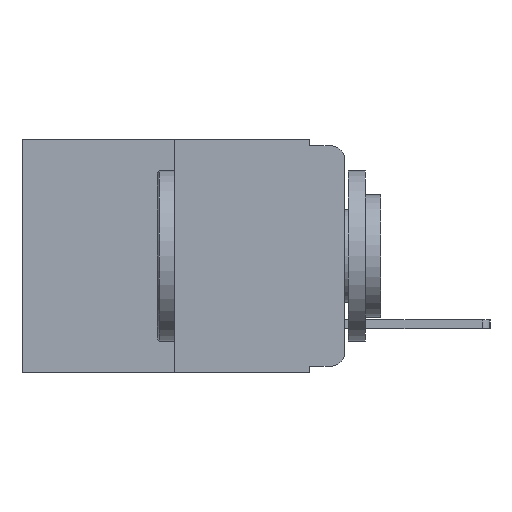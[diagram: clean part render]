
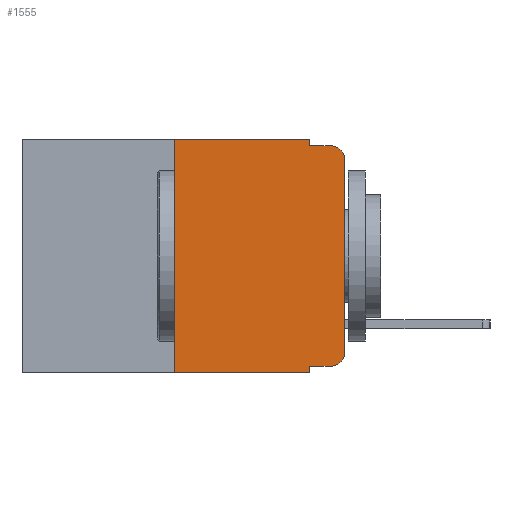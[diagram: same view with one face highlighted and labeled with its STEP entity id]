
A CAD part, left-side view. The second image highlights one B-rep face of the part: STEP entity #1555.
In plain terms, the highlighted planar face has unit normal (-1, 0, 0).
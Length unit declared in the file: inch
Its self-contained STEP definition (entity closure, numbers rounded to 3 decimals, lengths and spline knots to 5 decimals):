
#567 = AXIS2_PLACEMENT_3D ( 'NONE', #3577, #10929, #4782 ) ;
#870 = LINE ( 'NONE', #13710, #9405 ) ;
#1305 = LINE ( 'NONE', #6623, #4194 ) ;
#1432 = ORIENTED_EDGE ( 'NONE', *, *, #9063, .F. ) ;
#1555 = ADVANCED_FACE ( 'NONE', ( #7393 ), #8479, .F. ) ;
#1598 = VERTEX_POINT ( 'NONE', #12378 ) ;
#1655 = ORIENTED_EDGE ( 'NONE', *, *, #9168, .T. ) ;
#1799 = VERTEX_POINT ( 'NONE', #11805 ) ;
#1927 = CIRCLE ( 'NONE', #567, 0.02 ) ;
#2148 = LINE ( 'NONE', #9574, #10049 ) ;
#2835 = VECTOR ( 'NONE', #12388, 39.37008 ) ;
#3334 = CARTESIAN_POINT ( 'NONE',  ( 0., 0.051, -0.343 ) ) ;
#3475 = DIRECTION ( 'NONE',  ( 0., 0., -1. ) ) ;
#3577 = CARTESIAN_POINT ( 'NONE',  ( 0., 0.02, -0.313 ) ) ;
#3671 = DIRECTION ( 'NONE',  ( 0., 0., -1. ) ) ;
#3675 = DIRECTION ( 'NONE',  ( 1., 0., 0. ) ) ;
#4119 = CARTESIAN_POINT ( 'NONE',  ( 0., 0.473, 0. ) ) ;
#4194 = VECTOR ( 'NONE', #7621, 39.37008 ) ;
#4229 = CARTESIAN_POINT ( 'NONE',  ( 0., 0.051, 0. ) ) ;
#4305 = CARTESIAN_POINT ( 'NONE',  ( 0., 0.473, 0. ) ) ;
#4473 = CARTESIAN_POINT ( 'NONE',  ( 0., 0.02, -0.03 ) ) ;
#4632 = EDGE_CURVE ( 'NONE', #5760, #4680, #6195, .T. ) ;
#4680 = VERTEX_POINT ( 'NONE', #4229 ) ;
#4782 = DIRECTION ( 'NONE',  ( 0., 0., -1. ) ) ;
#4928 = CIRCLE ( 'NONE', #12534, 0.02 ) ;
#4971 = LINE ( 'NONE', #8127, #7082 ) ;
#5041 = VERTEX_POINT ( 'NONE', #12837 ) ;
#5429 = VECTOR ( 'NONE', #11841, 39.37008 ) ;
#5588 = DIRECTION ( 'NONE',  ( 0., 0., -1. ) ) ;
#5634 = DIRECTION ( 'NONE',  ( 0., 0., -1. ) ) ;
#5760 = VERTEX_POINT ( 'NONE', #13702 ) ;
#6060 = ORIENTED_EDGE ( 'NONE', *, *, #9047, .T. ) ;
#6081 = VECTOR ( 'NONE', #3475, 39.37008 ) ;
#6195 = LINE ( 'NONE', #4119, #2835 ) ;
#6409 = VECTOR ( 'NONE', #12736, 39.37008 ) ;
#6623 = CARTESIAN_POINT ( 'NONE',  ( 0., 0.051, -0.01 ) ) ;
#7048 = VERTEX_POINT ( 'NONE', #13305 ) ;
#7082 = VECTOR ( 'NONE', #9167, 39.37008 ) ;
#7393 = FACE_OUTER_BOUND ( 'NONE', #12363, .T. ) ;
#7621 = DIRECTION ( 'NONE',  ( 0., -1., 0. ) ) ;
#7659 = EDGE_CURVE ( 'NONE', #9181, #9071, #4971, .T. ) ;
#7700 = AXIS2_PLACEMENT_3D ( 'NONE', #4305, #3675, #3671 ) ;
#7748 = CARTESIAN_POINT ( 'NONE',  ( 0., 0.051, -0.333 ) ) ;
#7749 = ORIENTED_EDGE ( 'NONE', *, *, #7659, .T. ) ;
#8127 = CARTESIAN_POINT ( 'NONE',  ( 0., 0.473, -0.343 ) ) ;
#8351 = ORIENTED_EDGE ( 'NONE', *, *, #9111, .F. ) ;
#8479 = PLANE ( 'NONE',  #7700 ) ;
#9042 = EDGE_CURVE ( 'NONE', #1598, #5041, #2148, .T. ) ;
#9047 = EDGE_CURVE ( 'NONE', #5041, #7048, #4928, .T. ) ;
#9063 = EDGE_CURVE ( 'NONE', #11712, #7048, #1305, .T. ) ;
#9071 = VERTEX_POINT ( 'NONE', #3334 ) ;
#9111 = EDGE_CURVE ( 'NONE', #4680, #11712, #870, .T. ) ;
#9116 = EDGE_CURVE ( 'NONE', #9181, #5760, #11791, .T. ) ;
#9153 = ORIENTED_EDGE ( 'NONE', *, *, #9116, .F. ) ;
#9164 = EDGE_CURVE ( 'NONE', #13082, #9071, #13848, .T. ) ;
#9167 = DIRECTION ( 'NONE',  ( 0., -1., 0. ) ) ;
#9168 = EDGE_CURVE ( 'NONE', #13082, #1799, #11169, .T. ) ;
#9181 = VERTEX_POINT ( 'NONE', #13880 ) ;
#9233 = EDGE_CURVE ( 'NONE', #1799, #1598, #1927, .T. ) ;
#9405 = VECTOR ( 'NONE', #5634, 39.37008 ) ;
#9507 = ORIENTED_EDGE ( 'NONE', *, *, #9164, .F. ) ;
#9574 = CARTESIAN_POINT ( 'NONE',  ( 0., 0., 0. ) ) ;
#9796 = CARTESIAN_POINT ( 'NONE',  ( 0., 0.051, 0. ) ) ;
#10049 = VECTOR ( 'NONE', #12648, 39.37008 ) ;
#10929 = DIRECTION ( 'NONE',  ( -1., 0., 0. ) ) ;
#11169 = LINE ( 'NONE', #7748, #5429 ) ;
#11176 = CARTESIAN_POINT ( 'NONE',  ( 0., 0.051, -0.01 ) ) ;
#11512 = ORIENTED_EDGE ( 'NONE', *, *, #9233, .T. ) ;
#11671 = DIRECTION ( 'NONE',  ( -1., 0., 0. ) ) ;
#11712 = VERTEX_POINT ( 'NONE', #11176 ) ;
#11715 = CARTESIAN_POINT ( 'NONE',  ( 0., 0.25, 0. ) ) ;
#11760 = CARTESIAN_POINT ( 'NONE',  ( 0., 0.051, -0.333 ) ) ;
#11791 = LINE ( 'NONE', #11715, #6409 ) ;
#11805 = CARTESIAN_POINT ( 'NONE',  ( 0., 0.02, -0.333 ) ) ;
#11841 = DIRECTION ( 'NONE',  ( 0., -1., 0. ) ) ;
#12363 = EDGE_LOOP ( 'NONE', ( #13919, #6060, #1432, #8351, #13327, #9153, #7749, #9507, #1655, #11512 ) ) ;
#12378 = CARTESIAN_POINT ( 'NONE',  ( 0., 0., -0.313 ) ) ;
#12388 = DIRECTION ( 'NONE',  ( 0., -1., 0. ) ) ;
#12534 = AXIS2_PLACEMENT_3D ( 'NONE', #4473, #11671, #5588 ) ;
#12648 = DIRECTION ( 'NONE',  ( 0., 0., 1. ) ) ;
#12736 = DIRECTION ( 'NONE',  ( 0., 0., 1. ) ) ;
#12837 = CARTESIAN_POINT ( 'NONE',  ( 0., 0., -0.03 ) ) ;
#13082 = VERTEX_POINT ( 'NONE', #11760 ) ;
#13305 = CARTESIAN_POINT ( 'NONE',  ( 0., 0.02, -0.01 ) ) ;
#13327 = ORIENTED_EDGE ( 'NONE', *, *, #4632, .F. ) ;
#13702 = CARTESIAN_POINT ( 'NONE',  ( 0., 0.25, 0. ) ) ;
#13710 = CARTESIAN_POINT ( 'NONE',  ( 0., 0.051, 0. ) ) ;
#13848 = LINE ( 'NONE', #9796, #6081 ) ;
#13880 = CARTESIAN_POINT ( 'NONE',  ( 0., 0.25, -0.343 ) ) ;
#13919 = ORIENTED_EDGE ( 'NONE', *, *, #9042, .T. ) ;
